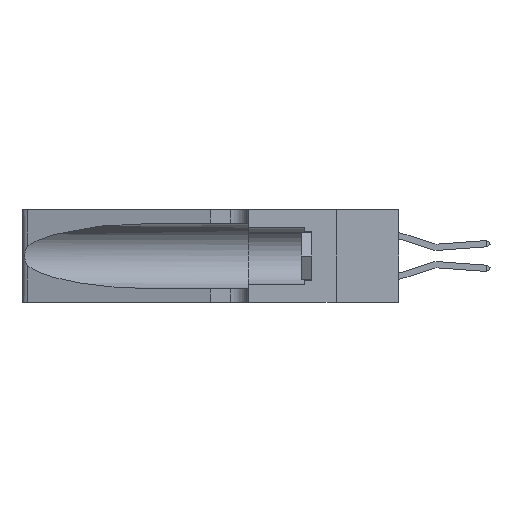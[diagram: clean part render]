
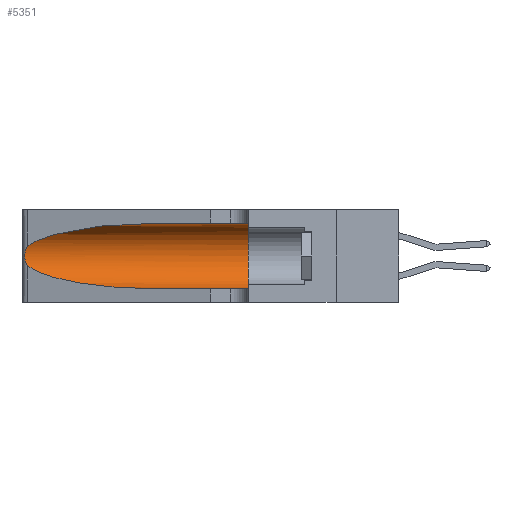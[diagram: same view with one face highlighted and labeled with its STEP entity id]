
A CAD part, left-side view. The second image highlights one B-rep face of the part: STEP entity #5351.
In plain terms, the highlighted cylindrical face has radius 3.308 mm (diameter 6.617 mm), a partial arc.
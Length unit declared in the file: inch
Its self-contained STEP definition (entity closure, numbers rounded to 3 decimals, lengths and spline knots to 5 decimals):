
#503 = VERTEX_POINT ( 'NONE', #8421 ) ;
#807 = CARTESIAN_POINT ( 'NONE',  ( 0.25487, 1.22718, 0.14631 ) ) ;
#992 = CARTESIAN_POINT ( 'NONE',  ( 0.25856, 1.23593, 0.16098 ) ) ;
#1143 = VERTEX_POINT ( 'NONE', #27306 ) ;
#1835 = EDGE_CURVE ( 'NONE', #1143, #5413, #24073, .T. ) ;
#2972 = CARTESIAN_POINT ( 'NONE',  ( 0.18966, 0.96281, 0.05475 ) ) ;
#3058 = CARTESIAN_POINT ( 'NONE',  ( 0.25487, 1.22718, 0.22369 ) ) ;
#3142 = CARTESIAN_POINT ( 'NONE',  ( 0.25639, 1.23186, 0.15144 ) ) ;
#3151 = VERTEX_POINT ( 'NONE', #23789 ) ;
#3477 = EDGE_CURVE ( 'NONE', #25258, #5413, #12202, .T. ) ;
#4675 = FACE_OUTER_BOUND ( 'NONE', #22041, .T. ) ;
#5287 = CARTESIAN_POINT ( 'NONE',  ( 0.25487, 1.22718, 0.14631 ) ) ;
#5351 = ADVANCED_FACE ( 'NONE', ( #4675 ), #15480, .F. ) ;
#5413 = VERTEX_POINT ( 'NONE', #9866 ) ;
#5703 = CARTESIAN_POINT ( 'NONE',  ( 0.1305, 1.61858, 0.05475 ) ) ;
#6190 = CARTESIAN_POINT ( 'NONE',  ( 0.1305, 0.72297, 0.31525 ) ) ;
#6456 = AXIS2_PLACEMENT_3D ( 'NONE', #9667, #24352, #20207 ) ;
#7391 = CARTESIAN_POINT ( 'NONE',  ( 0.25639, 1.23184, 0.21858 ) ) ;
#8384 = EDGE_CURVE ( 'NONE', #3151, #12799, #10347, .T. ) ;
#8394 = CARTESIAN_POINT ( 'NONE',  ( 0.1305, 0.35, 0.185 ) ) ;
#8421 = CARTESIAN_POINT ( 'NONE',  ( 0.1305, 0.72297, 0.31525 ) ) ;
#9602 = CARTESIAN_POINT ( 'NONE',  ( 0.25854, 1.2359, 0.20912 ) ) ;
#9667 = CARTESIAN_POINT ( 'NONE',  ( 0.1305, 1.61858, 0.185 ) ) ;
#9866 = CARTESIAN_POINT ( 'NONE',  ( 0.1305, 0.35, 0.05475 ) ) ;
#10347 = B_SPLINE_CURVE_WITH_KNOTS ( 'NONE', 3,
 ( #3058, #11659, #7391, #22213, #9602, #24281, #11755, #26335, #13899, #992, #16046, #3142, #18135, #5287 ),
 .UNSPECIFIED., .F., .F.,
 ( 4, 2, 2, 2, 2, 2, 4 ),
 ( 0., 0.00027, 0.00053, 0.00107, 0.0016, 0.00187, 0.00214 ),
 .UNSPECIFIED. ) ;
#10586 = DIRECTION ( 'NONE',  ( 0., 0., 1. ) ) ;
#10764 = VECTOR ( 'NONE', #18248, 39.37008 ) ;
#11554 = CARTESIAN_POINT ( 'NONE',  ( 0.1305, 0.72297, 0.05475 ) ) ;
#11583 = CARTESIAN_POINT ( 'NONE',  ( 0.2373, 1.15595, 0.08982 ) ) ;
#11659 = CARTESIAN_POINT ( 'NONE',  ( 0.25555, 1.22994, 0.2215 ) ) ;
#11755 = CARTESIAN_POINT ( 'NONE',  ( 0.26075, 1.23896, 0.19203 ) ) ;
#12159 = DIRECTION ( 'NONE',  ( 0., -1., 0. ) ) ;
#12202 = LINE ( 'NONE', #5703, #22699 ) ;
#12389 = AXIS2_PLACEMENT_3D ( 'NONE', #8394, #23142, #10586 ) ;
#12734 = CARTESIAN_POINT ( 'NONE',  ( 0.2373, 1.15595, 0.28018 ) ) ;
#12799 = VERTEX_POINT ( 'NONE', #25535 ) ;
#13249 =( BOUNDED_CURVE ( )  B_SPLINE_CURVE ( 3, ( #6190, #23156, #12734, #27287 ),
 .UNSPECIFIED., .F., .F. ) 
 B_SPLINE_CURVE_WITH_KNOTS ( ( 4, 4 ),
 ( 1.5708, 2.84003 ),
 .UNSPECIFIED. ) 
 CURVE ( )  GEOMETRIC_REPRESENTATION_ITEM ( )  RATIONAL_B_SPLINE_CURVE ( ( 1., 0.87, 0.87, 1. ) ) 
 REPRESENTATION_ITEM ( '' )  );
#13899 = CARTESIAN_POINT ( 'NONE',  ( 0.26017, 1.23833, 0.17102 ) ) ;
#15480 = CYLINDRICAL_SURFACE ( 'NONE', #6456, 0.13025 ) ;
#15510 = ORIENTED_EDGE ( 'NONE', *, *, #3477, .T. ) ;
#16046 = CARTESIAN_POINT ( 'NONE',  ( 0.25789, 1.23486, 0.15765 ) ) ;
#16424 = LINE ( 'NONE', #26443, #10764 ) ;
#17964 = CARTESIAN_POINT ( 'NONE',  ( 0.1305, 0.72297, 0.05475 ) ) ;
#18135 = CARTESIAN_POINT ( 'NONE',  ( 0.25555, 1.22993, 0.14849 ) ) ;
#18248 = DIRECTION ( 'NONE',  ( 0., -1., 0. ) ) ;
#18436 = EDGE_CURVE ( 'NONE', #503, #3151, #13249, .T. ) ;
#19370 = ORIENTED_EDGE ( 'NONE', *, *, #1835, .F. ) ;
#19680 = ORIENTED_EDGE ( 'NONE', *, *, #18436, .T. ) ;
#20120 = EDGE_CURVE ( 'NONE', #503, #1143, #16424, .T. ) ;
#20207 = DIRECTION ( 'NONE',  ( 0., 0., -1. ) ) ;
#20917 = ORIENTED_EDGE ( 'NONE', *, *, #20120, .F. ) ;
#20972 =( BOUNDED_CURVE ( )  B_SPLINE_CURVE ( 3, ( #807, #11583, #2972, #17964 ),
 .UNSPECIFIED., .F., .F. ) 
 B_SPLINE_CURVE_WITH_KNOTS ( ( 4, 4 ),
 ( 3.44316, 4.71239 ),
 .UNSPECIFIED. ) 
 CURVE ( )  GEOMETRIC_REPRESENTATION_ITEM ( )  RATIONAL_B_SPLINE_CURVE ( ( 1., 0.87, 0.87, 1. ) ) 
 REPRESENTATION_ITEM ( '' )  );
#21003 = ORIENTED_EDGE ( 'NONE', *, *, #22725, .T. ) ;
#21816 = ORIENTED_EDGE ( 'NONE', *, *, #8384, .T. ) ;
#22041 = EDGE_LOOP ( 'NONE', ( #19680, #21816, #21003, #15510, #19370, #20917 ) ) ;
#22213 = CARTESIAN_POINT ( 'NONE',  ( 0.25787, 1.23484, 0.2124 ) ) ;
#22699 = VECTOR ( 'NONE', #12159, 39.37008 ) ;
#22725 = EDGE_CURVE ( 'NONE', #12799, #25258, #20972, .T. ) ;
#23142 = DIRECTION ( 'NONE',  ( 0., 1., 0. ) ) ;
#23156 = CARTESIAN_POINT ( 'NONE',  ( 0.18966, 0.96281, 0.31525 ) ) ;
#23789 = CARTESIAN_POINT ( 'NONE',  ( 0.25487, 1.22718, 0.22369 ) ) ;
#24073 = CIRCLE ( 'NONE', #12389, 0.13025 ) ;
#24281 = CARTESIAN_POINT ( 'NONE',  ( 0.26018, 1.23835, 0.19895 ) ) ;
#24352 = DIRECTION ( 'NONE',  ( 0., -1., 0. ) ) ;
#25258 = VERTEX_POINT ( 'NONE', #11554 ) ;
#25535 = CARTESIAN_POINT ( 'NONE',  ( 0.25487, 1.22718, 0.14631 ) ) ;
#26335 = CARTESIAN_POINT ( 'NONE',  ( 0.26075, 1.23896, 0.178 ) ) ;
#26443 = CARTESIAN_POINT ( 'NONE',  ( 0.1305, 1.61858, 0.31525 ) ) ;
#27287 = CARTESIAN_POINT ( 'NONE',  ( 0.25487, 1.22718, 0.22369 ) ) ;
#27306 = CARTESIAN_POINT ( 'NONE',  ( 0.1305, 0.35, 0.31525 ) ) ;
